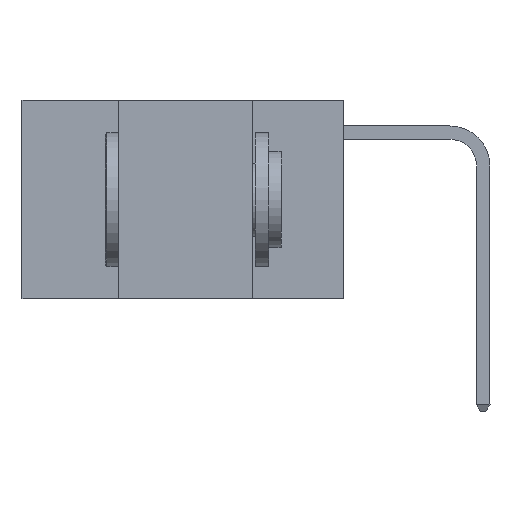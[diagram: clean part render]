
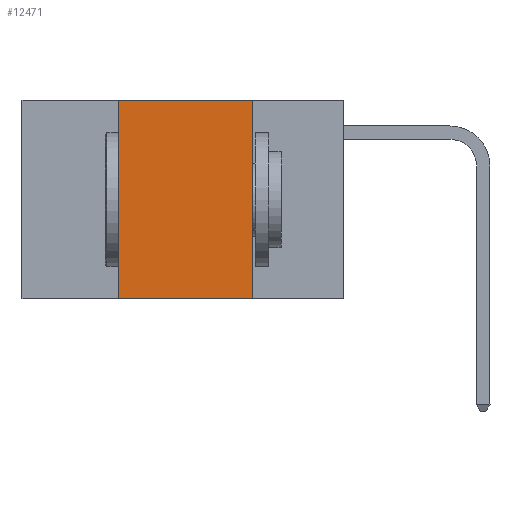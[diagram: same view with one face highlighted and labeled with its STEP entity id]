
A CAD part, left-side view. The second image highlights one B-rep face of the part: STEP entity #12471.
In plain terms, the highlighted planar face has unit normal (-1, 0, 0).
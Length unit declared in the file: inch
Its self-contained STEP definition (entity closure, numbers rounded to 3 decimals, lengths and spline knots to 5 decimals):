
#154 = VECTOR ( 'NONE', #3333, 39.37008 ) ;
#314 = CARTESIAN_POINT ( 'NONE',  ( 0., 0.6, 0. ) ) ;
#952 = LINE ( 'NONE', #10204, #10995 ) ;
#1055 = ORIENTED_EDGE ( 'NONE', *, *, #11707, .F. ) ;
#1169 = VECTOR ( 'NONE', #17306, 39.37008 ) ;
#2111 = DIRECTION ( 'NONE',  ( 0., 0., -1. ) ) ;
#2516 = VECTOR ( 'NONE', #15232, 39.37008 ) ;
#3089 = ORIENTED_EDGE ( 'NONE', *, *, #8388, .F. ) ;
#3333 = DIRECTION ( 'NONE',  ( 0., 0., 1. ) ) ;
#4271 = EDGE_CURVE ( 'NONE', #8412, #9998, #5278, .T. ) ;
#5124 = CARTESIAN_POINT ( 'NONE',  ( 0., 0.42, -0.37 ) ) ;
#5278 = LINE ( 'NONE', #7399, #1169 ) ;
#6769 = DIRECTION ( 'NONE',  ( 0., 0., -1. ) ) ;
#7399 = CARTESIAN_POINT ( 'NONE',  ( 0., 0.6, -0.37 ) ) ;
#7742 = EDGE_CURVE ( 'NONE', #8412, #8027, #13229, .T. ) ;
#7848 = ORIENTED_EDGE ( 'NONE', *, *, #4271, .T. ) ;
#8027 = VERTEX_POINT ( 'NONE', #12570 ) ;
#8071 = ORIENTED_EDGE ( 'NONE', *, *, #7742, .F. ) ;
#8388 = EDGE_CURVE ( 'NONE', #11989, #9998, #952, .T. ) ;
#8412 = VERTEX_POINT ( 'NONE', #5124 ) ;
#9135 = EDGE_LOOP ( 'NONE', ( #3089, #1055, #8071, #7848 ) ) ;
#9437 = AXIS2_PLACEMENT_3D ( 'NONE', #314, #12296, #2111 ) ;
#9998 = VERTEX_POINT ( 'NONE', #13875 ) ;
#10204 = CARTESIAN_POINT ( 'NONE',  ( 0., 0.17, 0. ) ) ;
#10649 = PLANE ( 'NONE',  #9437 ) ;
#10995 = VECTOR ( 'NONE', #6769, 39.37008 ) ;
#11707 = EDGE_CURVE ( 'NONE', #8027, #11989, #15896, .T. ) ;
#11989 = VERTEX_POINT ( 'NONE', #17468 ) ;
#12296 = DIRECTION ( 'NONE',  ( 1., 0., 0. ) ) ;
#12471 = ADVANCED_FACE ( 'NONE', ( #13591 ), #10649, .F. ) ;
#12570 = CARTESIAN_POINT ( 'NONE',  ( 0., 0.42, 0. ) ) ;
#13229 = LINE ( 'NONE', #15068, #154 ) ;
#13591 = FACE_OUTER_BOUND ( 'NONE', #9135, .T. ) ;
#13616 = CARTESIAN_POINT ( 'NONE',  ( 0., 0.6, 0. ) ) ;
#13875 = CARTESIAN_POINT ( 'NONE',  ( 0., 0.17, -0.37 ) ) ;
#15068 = CARTESIAN_POINT ( 'NONE',  ( 0., 0.42, 0. ) ) ;
#15232 = DIRECTION ( 'NONE',  ( 0., -1., 0. ) ) ;
#15896 = LINE ( 'NONE', #13616, #2516 ) ;
#17306 = DIRECTION ( 'NONE',  ( 0., -1., 0. ) ) ;
#17468 = CARTESIAN_POINT ( 'NONE',  ( 0., 0.17, 0. ) ) ;
